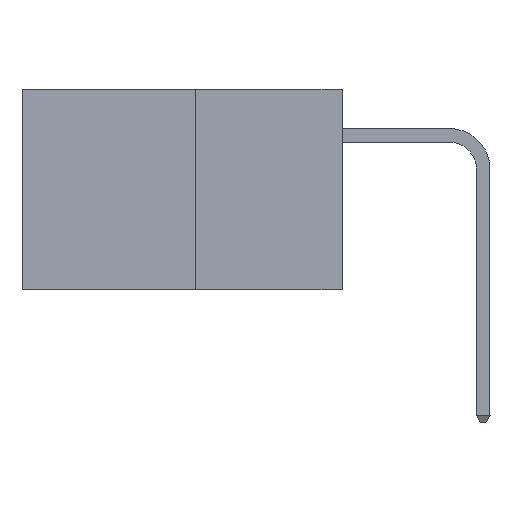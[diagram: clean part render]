
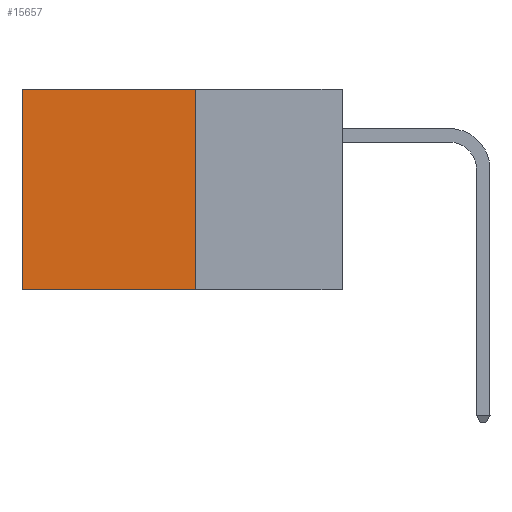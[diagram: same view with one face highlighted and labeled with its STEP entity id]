
A CAD part, left-side view. The second image highlights one B-rep face of the part: STEP entity #15657.
In plain terms, the highlighted planar face has unit normal (-1, 0, 0).
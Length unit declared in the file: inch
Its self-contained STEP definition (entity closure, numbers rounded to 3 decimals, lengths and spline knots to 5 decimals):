
#559 = LINE ( 'NONE', #9111, #5307 ) ;
#4845 = EDGE_CURVE ( 'NONE', #11172, #15774, #559, .T. ) ;
#5307 = VECTOR ( 'NONE', #22095, 39.37008 ) ;
#6255 = ORIENTED_EDGE ( 'NONE', *, *, #4845, .F. ) ;
#6324 = CARTESIAN_POINT ( 'NONE',  ( 0.277, 0.27, -0.37 ) ) ;
#6888 = VERTEX_POINT ( 'NONE', #27234 ) ;
#8180 = CARTESIAN_POINT ( 'NONE',  ( 0.277, 0.27, 0. ) ) ;
#8354 = DIRECTION ( 'NONE',  ( 1., 0., 0. ) ) ;
#8557 = ORIENTED_EDGE ( 'NONE', *, *, #9601, .T. ) ;
#9111 = CARTESIAN_POINT ( 'NONE',  ( 0.277, 0.27, -0.37 ) ) ;
#9601 = EDGE_CURVE ( 'NONE', #16899, #6888, #21690, .T. ) ;
#10938 = DIRECTION ( 'NONE',  ( 0., 0., -1. ) ) ;
#11074 = VECTOR ( 'NONE', #20403, 39.37008 ) ;
#11172 = VERTEX_POINT ( 'NONE', #19323 ) ;
#11496 = CARTESIAN_POINT ( 'NONE',  ( 0.277, 0.59, -0.37 ) ) ;
#11634 = VECTOR ( 'NONE', #10938, 39.37008 ) ;
#13269 = AXIS2_PLACEMENT_3D ( 'NONE', #21908, #8354, #24208 ) ;
#15076 = PLANE ( 'NONE',  #13269 ) ;
#15273 = CARTESIAN_POINT ( 'NONE',  ( 0.277, 0.59, -0.37 ) ) ;
#15657 = ADVANCED_FACE ( 'NONE', ( #19076 ), #15076, .F. ) ;
#15774 = VERTEX_POINT ( 'NONE', #15273 ) ;
#15977 = ORIENTED_EDGE ( 'NONE', *, *, #24431, .T. ) ;
#16899 = VERTEX_POINT ( 'NONE', #8180 ) ;
#17648 = LINE ( 'NONE', #6324, #11634 ) ;
#19076 = FACE_OUTER_BOUND ( 'NONE', #20233, .T. ) ;
#19323 = CARTESIAN_POINT ( 'NONE',  ( 0.277, 0.27, -0.37 ) ) ;
#20233 = EDGE_LOOP ( 'NONE', ( #15977, #6255, #29629, #8557 ) ) ;
#20403 = DIRECTION ( 'NONE',  ( 0., 1., 0. ) ) ;
#21366 = EDGE_CURVE ( 'NONE', #16899, #11172, #17648, .T. ) ;
#21690 = LINE ( 'NONE', #29483, #11074 ) ;
#21908 = CARTESIAN_POINT ( 'NONE',  ( 0.277, 0.27, -0.37 ) ) ;
#22043 = LINE ( 'NONE', #11496, #27401 ) ;
#22095 = DIRECTION ( 'NONE',  ( 0., 1., 0. ) ) ;
#24208 = DIRECTION ( 'NONE',  ( 0., 0., -1. ) ) ;
#24431 = EDGE_CURVE ( 'NONE', #6888, #15774, #22043, .T. ) ;
#25104 = DIRECTION ( 'NONE',  ( 0., 0., -1. ) ) ;
#27234 = CARTESIAN_POINT ( 'NONE',  ( 0.277, 0.59, 0. ) ) ;
#27401 = VECTOR ( 'NONE', #25104, 39.37008 ) ;
#29483 = CARTESIAN_POINT ( 'NONE',  ( 0.277, 0.27, 0. ) ) ;
#29629 = ORIENTED_EDGE ( 'NONE', *, *, #21366, .F. ) ;
